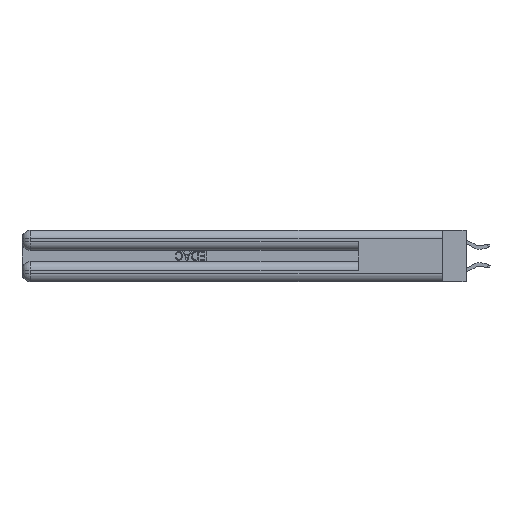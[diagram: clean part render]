
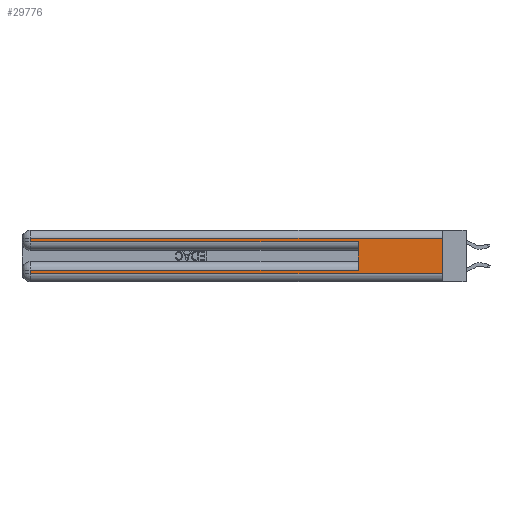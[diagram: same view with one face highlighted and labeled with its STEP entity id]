
A CAD part, left-side view. The second image highlights one B-rep face of the part: STEP entity #29776.
In plain terms, the highlighted planar face has unit normal (-1, 0, 0).
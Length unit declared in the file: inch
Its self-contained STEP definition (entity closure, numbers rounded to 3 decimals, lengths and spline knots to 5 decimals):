
#84 = VECTOR ( 'NONE', #7654, 39.37008 ) ;
#208 = VECTOR ( 'NONE', #7796, 39.37008 ) ;
#373 = DIRECTION ( 'NONE',  ( 0., -1., 0. ) ) ;
#420 = CARTESIAN_POINT ( 'NONE',  ( 0., 0.6, 0.145 ) ) ;
#743 = VERTEX_POINT ( 'NONE', #26974 ) ;
#1013 = CARTESIAN_POINT ( 'NONE',  ( 0., 2.94, 0.085 ) ) ;
#1097 = EDGE_CURVE ( 'NONE', #743, #20433, #2185, .T. ) ;
#1320 = VECTOR ( 'NONE', #16177, 39.37008 ) ;
#1526 = CARTESIAN_POINT ( 'NONE',  ( 0., 0., 0.06 ) ) ;
#1686 = EDGE_LOOP ( 'NONE', ( #9862, #25484, #28475, #19373, #28228, #6480, #22335, #30000 ) ) ;
#2185 = LINE ( 'NONE', #22186, #5695 ) ;
#3278 = DIRECTION ( 'NONE',  ( 1., 0., 0. ) ) ;
#3906 = EDGE_CURVE ( 'NONE', #21856, #17536, #15657, .T. ) ;
#5395 = VECTOR ( 'NONE', #373, 39.37008 ) ;
#5695 = VECTOR ( 'NONE', #31527, 39.37008 ) ;
#5706 = EDGE_CURVE ( 'NONE', #21043, #26325, #6323, .T. ) ;
#5731 = CARTESIAN_POINT ( 'NONE',  ( 0., 0., 0.37 ) ) ;
#6323 = LINE ( 'NONE', #11571, #1320 ) ;
#6480 = ORIENTED_EDGE ( 'NONE', *, *, #19682, .T. ) ;
#7654 = DIRECTION ( 'NONE',  ( 0., 1., 0. ) ) ;
#7796 = DIRECTION ( 'NONE',  ( 0., 0., -1. ) ) ;
#8188 = EDGE_CURVE ( 'NONE', #14631, #743, #16343, .T. ) ;
#8568 = LINE ( 'NONE', #23487, #29297 ) ;
#8590 = DIRECTION ( 'NONE',  ( 0., 0., 1. ) ) ;
#9292 = CARTESIAN_POINT ( 'NONE',  ( 0., 2.94, 0.37 ) ) ;
#9862 = ORIENTED_EDGE ( 'NONE', *, *, #17863, .F. ) ;
#10275 = CARTESIAN_POINT ( 'NONE',  ( 0., 2.94, 0.285 ) ) ;
#10772 = AXIS2_PLACEMENT_3D ( 'NONE', #5731, #3278, #28823 ) ;
#11345 = VERTEX_POINT ( 'NONE', #10275 ) ;
#11571 = CARTESIAN_POINT ( 'NONE',  ( 0., 0., 0.31 ) ) ;
#12076 = LINE ( 'NONE', #23059, #84 ) ;
#14335 = VECTOR ( 'NONE', #8590, 39.37008 ) ;
#14631 = VERTEX_POINT ( 'NONE', #1013 ) ;
#15657 = LINE ( 'NONE', #420, #14335 ) ;
#16070 = CARTESIAN_POINT ( 'NONE',  ( 0., 0.6, 0.285 ) ) ;
#16177 = DIRECTION ( 'NONE',  ( 0., 1., 0. ) ) ;
#16343 = LINE ( 'NONE', #9292, #21537 ) ;
#17536 = VERTEX_POINT ( 'NONE', #16070 ) ;
#17863 = EDGE_CURVE ( 'NONE', #21043, #20433, #8568, .T. ) ;
#18106 = LINE ( 'NONE', #28092, #208 ) ;
#18138 = CARTESIAN_POINT ( 'NONE',  ( 0., 0., 0.31 ) ) ;
#18199 = FACE_OUTER_BOUND ( 'NONE', #1686, .T. ) ;
#19373 = ORIENTED_EDGE ( 'NONE', *, *, #26507, .T. ) ;
#19682 = EDGE_CURVE ( 'NONE', #21856, #14631, #12076, .T. ) ;
#20362 = CARTESIAN_POINT ( 'NONE',  ( 0., 0., 0.285 ) ) ;
#20433 = VERTEX_POINT ( 'NONE', #1526 ) ;
#21043 = VERTEX_POINT ( 'NONE', #18138 ) ;
#21349 = DIRECTION ( 'NONE',  ( 0., 0., -1. ) ) ;
#21537 = VECTOR ( 'NONE', #28946, 39.37008 ) ;
#21856 = VERTEX_POINT ( 'NONE', #31127 ) ;
#22186 = CARTESIAN_POINT ( 'NONE',  ( 0., 0., 0.06 ) ) ;
#22335 = ORIENTED_EDGE ( 'NONE', *, *, #8188, .T. ) ;
#23059 = CARTESIAN_POINT ( 'NONE',  ( 0., 0., 0.085 ) ) ;
#23487 = CARTESIAN_POINT ( 'NONE',  ( 0., 0., 0.37 ) ) ;
#24304 = CARTESIAN_POINT ( 'NONE',  ( 0., 2.94, 0.31 ) ) ;
#25484 = ORIENTED_EDGE ( 'NONE', *, *, #5706, .T. ) ;
#26325 = VERTEX_POINT ( 'NONE', #24304 ) ;
#26507 = EDGE_CURVE ( 'NONE', #11345, #17536, #27886, .T. ) ;
#26974 = CARTESIAN_POINT ( 'NONE',  ( 0., 2.94, 0.06 ) ) ;
#27402 = EDGE_CURVE ( 'NONE', #26325, #11345, #18106, .T. ) ;
#27886 = LINE ( 'NONE', #20362, #5395 ) ;
#28092 = CARTESIAN_POINT ( 'NONE',  ( 0., 2.94, 0.37 ) ) ;
#28228 = ORIENTED_EDGE ( 'NONE', *, *, #3906, .F. ) ;
#28340 = PLANE ( 'NONE',  #10772 ) ;
#28475 = ORIENTED_EDGE ( 'NONE', *, *, #27402, .T. ) ;
#28823 = DIRECTION ( 'NONE',  ( 0., 0., -1. ) ) ;
#28946 = DIRECTION ( 'NONE',  ( 0., 0., -1. ) ) ;
#29297 = VECTOR ( 'NONE', #21349, 39.37008 ) ;
#29776 = ADVANCED_FACE ( 'NONE', ( #18199 ), #28340, .F. ) ;
#30000 = ORIENTED_EDGE ( 'NONE', *, *, #1097, .T. ) ;
#31127 = CARTESIAN_POINT ( 'NONE',  ( 0., 0.6, 0.085 ) ) ;
#31527 = DIRECTION ( 'NONE',  ( 0., -1., 0. ) ) ;
